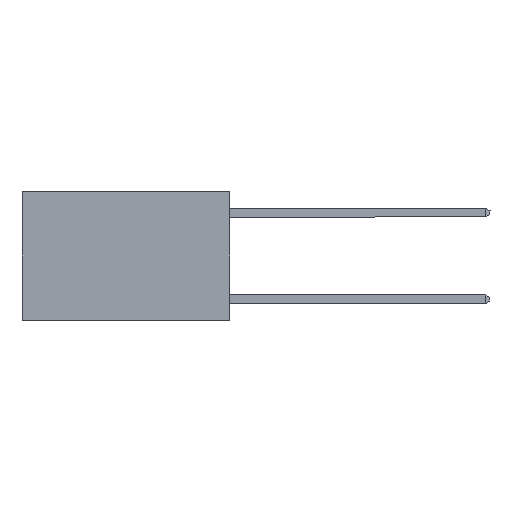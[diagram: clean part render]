
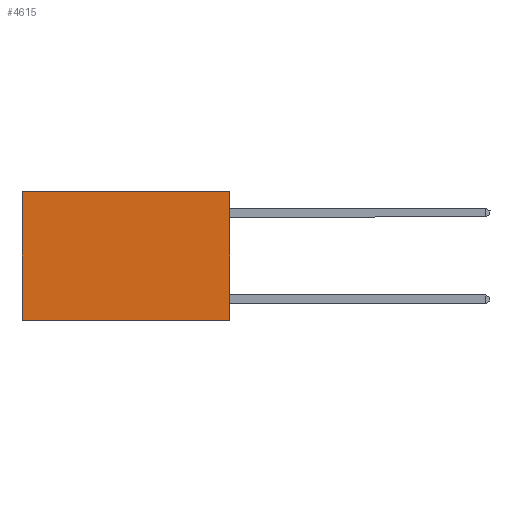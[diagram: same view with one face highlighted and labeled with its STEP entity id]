
A CAD part, left-side view. The second image highlights one B-rep face of the part: STEP entity #4615.
In plain terms, the highlighted planar face has unit normal (-1, 0, 0).
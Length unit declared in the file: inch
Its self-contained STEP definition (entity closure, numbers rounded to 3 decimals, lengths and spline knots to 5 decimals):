
#586 = EDGE_CURVE ( 'NONE', #5631, #4996, #9910, .T. ) ;
#848 = DIRECTION ( 'NONE',  ( 0., 0., -1. ) ) ;
#1034 = CARTESIAN_POINT ( 'NONE',  ( 0.2625, 0., -0.37 ) ) ;
#1401 = DIRECTION ( 'NONE',  ( 0., 0., -1. ) ) ;
#1608 = CARTESIAN_POINT ( 'NONE',  ( 0.2625, 0.6, 0. ) ) ;
#1852 = DIRECTION ( 'NONE',  ( 0., 1., 0. ) ) ;
#1872 = EDGE_LOOP ( 'NONE', ( #3772, #3796, #3804, #3828 ) ) ;
#1966 = CARTESIAN_POINT ( 'NONE',  ( 0.2625, 0., 0. ) ) ;
#2101 = VECTOR ( 'NONE', #7242, 39.37008 ) ;
#2337 = EDGE_CURVE ( 'NONE', #4104, #5631, #9865, .T. ) ;
#2628 = VECTOR ( 'NONE', #6171, 39.37008 ) ;
#2821 = CARTESIAN_POINT ( 'NONE',  ( 0.2625, 0., 0. ) ) ;
#3772 = ORIENTED_EDGE ( 'NONE', *, *, #586, .T. ) ;
#3796 = ORIENTED_EDGE ( 'NONE', *, *, #10004, .F. ) ;
#3804 = ORIENTED_EDGE ( 'NONE', *, *, #9173, .F. ) ;
#3828 = ORIENTED_EDGE ( 'NONE', *, *, #2337, .T. ) ;
#3941 = FACE_OUTER_BOUND ( 'NONE', #1872, .T. ) ;
#4104 = VERTEX_POINT ( 'NONE', #2821 ) ;
#4472 = LINE ( 'NONE', #1966, #2101 ) ;
#4615 = ADVANCED_FACE ( 'NONE', ( #3941 ), #10520, .F. ) ;
#4769 = AXIS2_PLACEMENT_3D ( 'NONE', #10489, #6632, #1401 ) ;
#4801 = CARTESIAN_POINT ( 'NONE',  ( 0.2625, 0.6, 0. ) ) ;
#4996 = VERTEX_POINT ( 'NONE', #8449 ) ;
#5468 = VECTOR ( 'NONE', #848, 39.37008 ) ;
#5631 = VERTEX_POINT ( 'NONE', #1608 ) ;
#6111 = CARTESIAN_POINT ( 'NONE',  ( 0.2625, 0., 0. ) ) ;
#6171 = DIRECTION ( 'NONE',  ( 0., 1., 0. ) ) ;
#6632 = DIRECTION ( 'NONE',  ( 1., 0., 0. ) ) ;
#7242 = DIRECTION ( 'NONE',  ( 0., 0., -1. ) ) ;
#7483 = CARTESIAN_POINT ( 'NONE',  ( 0.2625, 0., -0.37 ) ) ;
#7908 = LINE ( 'NONE', #1034, #9375 ) ;
#8449 = CARTESIAN_POINT ( 'NONE',  ( 0.2625, 0.6, -0.37 ) ) ;
#8521 = VERTEX_POINT ( 'NONE', #7483 ) ;
#9173 = EDGE_CURVE ( 'NONE', #4104, #8521, #4472, .T. ) ;
#9375 = VECTOR ( 'NONE', #1852, 39.37008 ) ;
#9865 = LINE ( 'NONE', #6111, #2628 ) ;
#9910 = LINE ( 'NONE', #4801, #5468 ) ;
#10004 = EDGE_CURVE ( 'NONE', #8521, #4996, #7908, .T. ) ;
#10489 = CARTESIAN_POINT ( 'NONE',  ( 0.2625, 0., 0. ) ) ;
#10520 = PLANE ( 'NONE',  #4769 ) ;
